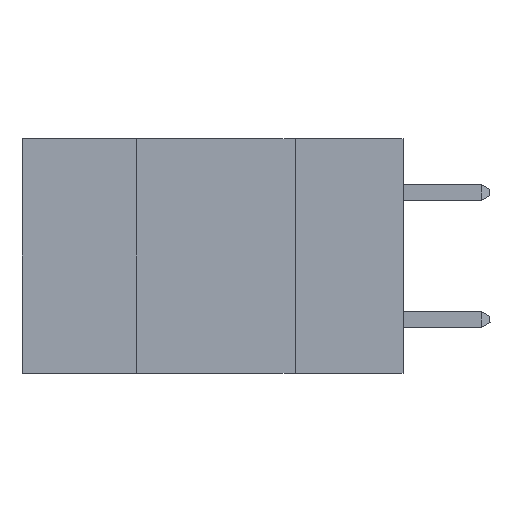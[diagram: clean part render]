
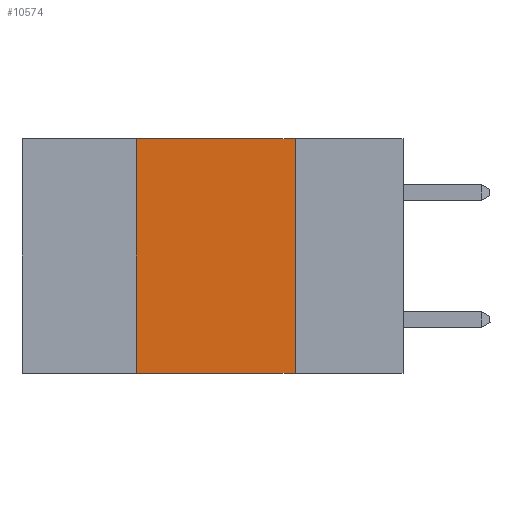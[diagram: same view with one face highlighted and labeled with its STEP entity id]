
A CAD part, left-side view. The second image highlights one B-rep face of the part: STEP entity #10574.
In plain terms, the highlighted planar face has unit normal (-1, 0, 0).
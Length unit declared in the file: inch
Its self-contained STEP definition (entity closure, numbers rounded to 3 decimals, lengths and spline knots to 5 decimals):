
#83 = ORIENTED_EDGE ( 'NONE', *, *, #9937, .F. ) ;
#160 = EDGE_CURVE ( 'NONE', #8337, #6024, #2164, .T. ) ;
#549 = CARTESIAN_POINT ( 'NONE',  ( 0., 0.17, 0. ) ) ;
#588 = ORIENTED_EDGE ( 'NONE', *, *, #160, .T. ) ;
#843 = FACE_OUTER_BOUND ( 'NONE', #9321, .T. ) ;
#1597 = CARTESIAN_POINT ( 'NONE',  ( 0., 0.6, 0. ) ) ;
#1705 = EDGE_CURVE ( 'NONE', #8337, #3691, #10111, .T. ) ;
#1859 = VECTOR ( 'NONE', #6535, 39.37008 ) ;
#2164 = LINE ( 'NONE', #8138, #7538 ) ;
#2181 = CARTESIAN_POINT ( 'NONE',  ( 0., 0.42, 0. ) ) ;
#2510 = LINE ( 'NONE', #4206, #10056 ) ;
#3425 = DIRECTION ( 'NONE',  ( 0., 0., -1. ) ) ;
#3691 = VERTEX_POINT ( 'NONE', #7492 ) ;
#4206 = CARTESIAN_POINT ( 'NONE',  ( 0., 0.17, 0. ) ) ;
#5159 = DIRECTION ( 'NONE',  ( 1., 0., 0. ) ) ;
#6024 = VERTEX_POINT ( 'NONE', #11311 ) ;
#6535 = DIRECTION ( 'NONE',  ( 0., 0., 1. ) ) ;
#7463 = VECTOR ( 'NONE', #10083, 39.37008 ) ;
#7492 = CARTESIAN_POINT ( 'NONE',  ( 0., 0.42, 0. ) ) ;
#7538 = VECTOR ( 'NONE', #10842, 39.37008 ) ;
#7645 = ORIENTED_EDGE ( 'NONE', *, *, #7850, .F. ) ;
#7850 = EDGE_CURVE ( 'NONE', #10913, #6024, #2510, .T. ) ;
#8138 = CARTESIAN_POINT ( 'NONE',  ( 0., 0.6, -0.37 ) ) ;
#8164 = CARTESIAN_POINT ( 'NONE',  ( 0., 0.42, -0.37 ) ) ;
#8181 = LINE ( 'NONE', #8239, #7463 ) ;
#8239 = CARTESIAN_POINT ( 'NONE',  ( 0., 0.6, 0. ) ) ;
#8337 = VERTEX_POINT ( 'NONE', #8164 ) ;
#8678 = DIRECTION ( 'NONE',  ( 0., 0., -1. ) ) ;
#8915 = ORIENTED_EDGE ( 'NONE', *, *, #1705, .F. ) ;
#9321 = EDGE_LOOP ( 'NONE', ( #7645, #83, #8915, #588 ) ) ;
#9543 = PLANE ( 'NONE',  #10594 ) ;
#9937 = EDGE_CURVE ( 'NONE', #3691, #10913, #8181, .T. ) ;
#10056 = VECTOR ( 'NONE', #3425, 39.37008 ) ;
#10083 = DIRECTION ( 'NONE',  ( 0., -1., 0. ) ) ;
#10111 = LINE ( 'NONE', #2181, #1859 ) ;
#10574 = ADVANCED_FACE ( 'NONE', ( #843 ), #9543, .F. ) ;
#10594 = AXIS2_PLACEMENT_3D ( 'NONE', #1597, #5159, #8678 ) ;
#10842 = DIRECTION ( 'NONE',  ( 0., -1., 0. ) ) ;
#10913 = VERTEX_POINT ( 'NONE', #549 ) ;
#11311 = CARTESIAN_POINT ( 'NONE',  ( 0., 0.17, -0.37 ) ) ;
